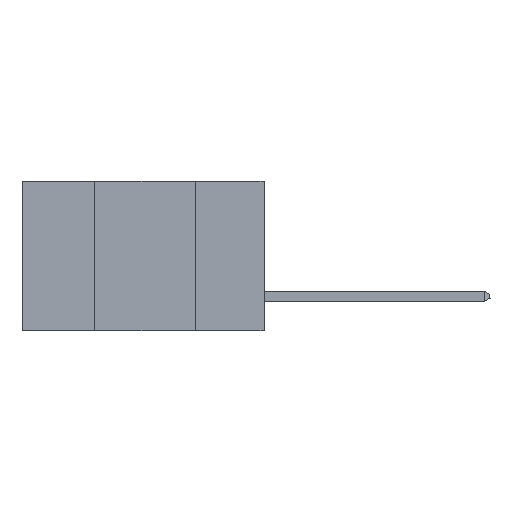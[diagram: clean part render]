
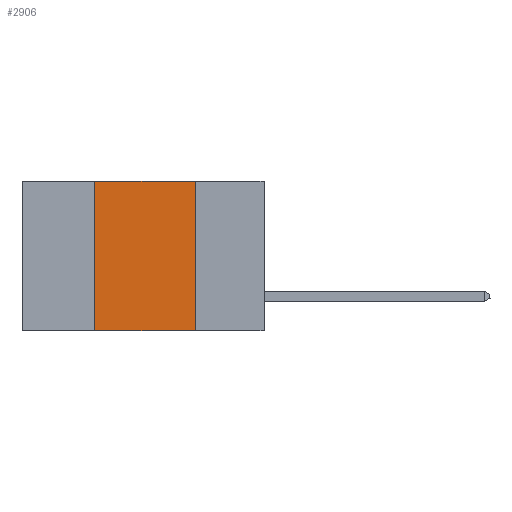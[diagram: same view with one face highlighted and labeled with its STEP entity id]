
A CAD part, left-side view. The second image highlights one B-rep face of the part: STEP entity #2906.
In plain terms, the highlighted planar face has unit normal (-1, 0, 0).
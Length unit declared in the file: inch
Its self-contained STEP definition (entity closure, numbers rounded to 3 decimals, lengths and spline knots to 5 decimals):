
#154 = PLANE ( 'NONE',  #5629 ) ;
#377 = VECTOR ( 'NONE', #6881, 39.37008 ) ;
#501 = EDGE_CURVE ( 'NONE', #16267, #12255, #1565, .T. ) ;
#894 = VECTOR ( 'NONE', #15781, 39.37008 ) ;
#1565 = LINE ( 'NONE', #15650, #894 ) ;
#1790 = LINE ( 'NONE', #14236, #377 ) ;
#2906 = ADVANCED_FACE ( 'NONE', ( #13216 ), #154, .F. ) ;
#3616 = CARTESIAN_POINT ( 'NONE',  ( 0., 0.17, 0. ) ) ;
#4721 = CARTESIAN_POINT ( 'NONE',  ( 0., 0.42, 0. ) ) ;
#5629 = AXIS2_PLACEMENT_3D ( 'NONE', #10565, #14832, #5996 ) ;
#5996 = DIRECTION ( 'NONE',  ( 0., 0., -1. ) ) ;
#6881 = DIRECTION ( 'NONE',  ( 0., -1., 0. ) ) ;
#8529 = ORIENTED_EDGE ( 'NONE', *, *, #10392, .F. ) ;
#9267 = CARTESIAN_POINT ( 'NONE',  ( 0., 0.17, -0.37 ) ) ;
#9272 = VECTOR ( 'NONE', #10704, 39.37008 ) ;
#10392 = EDGE_CURVE ( 'NONE', #12255, #15074, #11261, .T. ) ;
#10565 = CARTESIAN_POINT ( 'NONE',  ( 0., 0.6, 0. ) ) ;
#10704 = DIRECTION ( 'NONE',  ( 0., 0., 1. ) ) ;
#10822 = EDGE_LOOP ( 'NONE', ( #8529, #17642, #17771, #12644 ) ) ;
#11261 = LINE ( 'NONE', #13318, #16788 ) ;
#11646 = CARTESIAN_POINT ( 'NONE',  ( 0., 0.42, -0.37 ) ) ;
#12255 = VERTEX_POINT ( 'NONE', #3616 ) ;
#12397 = EDGE_CURVE ( 'NONE', #15491, #15074, #1790, .T. ) ;
#12644 = ORIENTED_EDGE ( 'NONE', *, *, #12397, .T. ) ;
#13216 = FACE_OUTER_BOUND ( 'NONE', #10822, .T. ) ;
#13318 = CARTESIAN_POINT ( 'NONE',  ( 0., 0.17, 0. ) ) ;
#13947 = EDGE_CURVE ( 'NONE', #15491, #16267, #15058, .T. ) ;
#14236 = CARTESIAN_POINT ( 'NONE',  ( 0., 0.6, -0.37 ) ) ;
#14789 = DIRECTION ( 'NONE',  ( 0., 0., -1. ) ) ;
#14832 = DIRECTION ( 'NONE',  ( 1., 0., 0. ) ) ;
#15058 = LINE ( 'NONE', #15157, #9272 ) ;
#15074 = VERTEX_POINT ( 'NONE', #9267 ) ;
#15157 = CARTESIAN_POINT ( 'NONE',  ( 0., 0.42, 0. ) ) ;
#15491 = VERTEX_POINT ( 'NONE', #11646 ) ;
#15650 = CARTESIAN_POINT ( 'NONE',  ( 0., 0.6, 0. ) ) ;
#15781 = DIRECTION ( 'NONE',  ( 0., -1., 0. ) ) ;
#16267 = VERTEX_POINT ( 'NONE', #4721 ) ;
#16788 = VECTOR ( 'NONE', #14789, 39.37008 ) ;
#17642 = ORIENTED_EDGE ( 'NONE', *, *, #501, .F. ) ;
#17771 = ORIENTED_EDGE ( 'NONE', *, *, #13947, .F. ) ;
